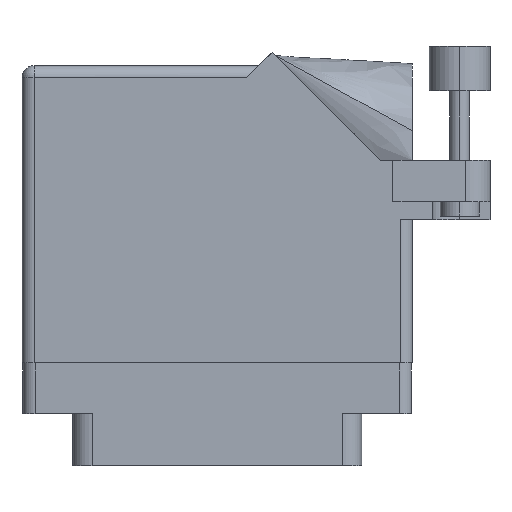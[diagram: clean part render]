
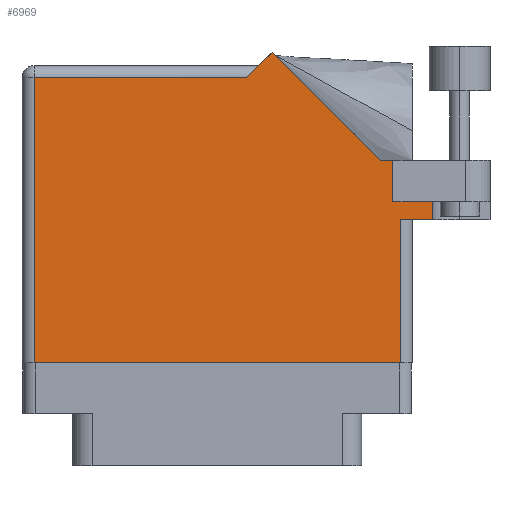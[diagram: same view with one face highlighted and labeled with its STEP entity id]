
A CAD part, front view. The second image highlights one B-rep face of the part: STEP entity #6969.
In plain terms, the highlighted face is planar.
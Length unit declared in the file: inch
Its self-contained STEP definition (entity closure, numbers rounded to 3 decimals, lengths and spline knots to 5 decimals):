
#476 = CARTESIAN_POINT ( 'NONE',  ( 2.1115, 1.16177, 0. ) ) ;
#520 = DIRECTION ( 'NONE',  ( 0., 1., 0. ) ) ;
#917 = CARTESIAN_POINT ( 'NONE',  ( 1.217, 1.53, 0. ) ) ;
#1288 = ORIENTED_EDGE ( 'NONE', *, *, #13473, .T. ) ;
#1426 = VECTOR ( 'NONE', #3656, 39.37008 ) ;
#2371 = ORIENTED_EDGE ( 'NONE', *, *, #24160, .T. ) ;
#2692 = VERTEX_POINT ( 'NONE', #9804 ) ;
#2951 = LINE ( 'NONE', #38883, #31933 ) ;
#3011 = DIRECTION ( 'NONE',  ( 1., 0., 0. ) ) ;
#3620 = VERTEX_POINT ( 'NONE', #18843 ) ;
#3656 = DIRECTION ( 'NONE',  ( -0.707, -0.707, 0. ) ) ;
#3920 = CARTESIAN_POINT ( 'NONE',  ( 1.84442, 1.044, 0. ) ) ;
#4170 = LINE ( 'NONE', #12082, #34573 ) ;
#4272 = VERTEX_POINT ( 'NONE', #17402 ) ;
#4332 = ORIENTED_EDGE ( 'NONE', *, *, #19496, .T. ) ;
#4532 = VECTOR ( 'NONE', #7852, 39.37008 ) ;
#5085 = EDGE_CURVE ( 'NONE', #17745, #25704, #18032, .T. ) ;
#6712 = VECTOR ( 'NONE', #9909, 39.37008 ) ;
#6969 = ADVANCED_FACE ( 'NONE', ( #23061 ), #28050, .F. ) ;
#7198 = ORIENTED_EDGE ( 'NONE', *, *, #5085, .T. ) ;
#7803 = CARTESIAN_POINT ( 'NONE',  ( 1.84442, 1.044, 0. ) ) ;
#7852 = DIRECTION ( 'NONE',  ( -1., 0., 0. ) ) ;
#8008 = DIRECTION ( 'NONE',  ( 0., -1., 0. ) ) ;
#8242 = EDGE_CURVE ( 'NONE', #23739, #4272, #24572, .T. ) ;
#9316 = VERTEX_POINT ( 'NONE', #32842 ) ;
#9490 = CARTESIAN_POINT ( 'NONE',  ( 0., 1.53, 0. ) ) ;
#9804 = CARTESIAN_POINT ( 'NONE',  ( 1.948, 0., 0. ) ) ;
#9883 = DIRECTION ( 'NONE',  ( 0., 0., -1. ) ) ;
#9909 = DIRECTION ( 'NONE',  ( 1., 0., 0. ) ) ;
#9930 = VECTOR ( 'NONE', #29068, 39.37008 ) ;
#10532 = CARTESIAN_POINT ( 'NONE',  ( 1.28771, 1.60071, 0. ) ) ;
#10705 = CARTESIAN_POINT ( 'NONE',  ( 0.062, 1.468, 0. ) ) ;
#11005 = ORIENTED_EDGE ( 'NONE', *, *, #18687, .F. ) ;
#11938 = VERTEX_POINT ( 'NONE', #29782 ) ;
#12082 = CARTESIAN_POINT ( 'NONE',  ( 1.91, 0.831, 0. ) ) ;
#12154 = ORIENTED_EDGE ( 'NONE', *, *, #19213, .T. ) ;
#12730 = LINE ( 'NONE', #22027, #35997 ) ;
#13073 = CARTESIAN_POINT ( 'NONE',  ( 2.01, 0.737, 0. ) ) ;
#13217 = CARTESIAN_POINT ( 'NONE',  ( 2.1115, 0.831, 0. ) ) ;
#13473 = EDGE_CURVE ( 'NONE', #11938, #17745, #15976, .T. ) ;
#14823 = DIRECTION ( 'NONE',  ( -1., 0., 0. ) ) ;
#15074 = ORIENTED_EDGE ( 'NONE', *, *, #16124, .T. ) ;
#15083 = LINE ( 'NONE', #32227, #33104 ) ;
#15620 = DIRECTION ( 'NONE',  ( 0., -1., 0. ) ) ;
#15976 = LINE ( 'NONE', #38513, #4532 ) ;
#16124 = EDGE_CURVE ( 'NONE', #2692, #9316, #2951, .T. ) ;
#16677 = EDGE_CURVE ( 'NONE', #30541, #2692, #30990, .T. ) ;
#16974 = VERTEX_POINT ( 'NONE', #10705 ) ;
#17124 = LINE ( 'NONE', #917, #1426 ) ;
#17402 = CARTESIAN_POINT ( 'NONE',  ( 2.1115, 0.737, 0. ) ) ;
#17731 = EDGE_CURVE ( 'NONE', #25704, #3620, #17124, .T. ) ;
#17745 = VERTEX_POINT ( 'NONE', #3920 ) ;
#17789 = LINE ( 'NONE', #13073, #22056 ) ;
#18032 = LINE ( 'NONE', #7803, #9930 ) ;
#18687 = EDGE_CURVE ( 'NONE', #32509, #23739, #4170, .T. ) ;
#18833 = EDGE_CURVE ( 'NONE', #32509, #11938, #12730, .T. ) ;
#18843 = CARTESIAN_POINT ( 'NONE',  ( 1.155, 1.468, 0. ) ) ;
#19213 = EDGE_CURVE ( 'NONE', #16974, #30541, #36444, .T. ) ;
#19496 = EDGE_CURVE ( 'NONE', #3620, #16974, #15083, .T. ) ;
#20102 = CARTESIAN_POINT ( 'NONE',  ( 0.062, 0., 0. ) ) ;
#20828 = ORIENTED_EDGE ( 'NONE', *, *, #8242, .F. ) ;
#22027 = CARTESIAN_POINT ( 'NONE',  ( 1.91, 0.831, 0. ) ) ;
#22056 = VECTOR ( 'NONE', #27670, 39.37008 ) ;
#23061 = FACE_OUTER_BOUND ( 'NONE', #38602, .T. ) ;
#23434 = CARTESIAN_POINT ( 'NONE',  ( 1.91, 0.831, 0. ) ) ;
#23739 = VERTEX_POINT ( 'NONE', #13217 ) ;
#24160 = EDGE_CURVE ( 'NONE', #9316, #4272, #17789, .T. ) ;
#24572 = LINE ( 'NONE', #476, #31721 ) ;
#24575 = VECTOR ( 'NONE', #8008, 39.37008 ) ;
#24699 = ORIENTED_EDGE ( 'NONE', *, *, #18833, .T. ) ;
#25704 = VERTEX_POINT ( 'NONE', #10532 ) ;
#26702 = DIRECTION ( 'NONE',  ( 0., 1., 0. ) ) ;
#27670 = DIRECTION ( 'NONE',  ( 1., 0., 0. ) ) ;
#27754 = CARTESIAN_POINT ( 'NONE',  ( 0.062, 0., 0. ) ) ;
#28050 = PLANE ( 'NONE',  #33389 ) ;
#29068 = DIRECTION ( 'NONE',  ( -0.707, 0.707, 0. ) ) ;
#29782 = CARTESIAN_POINT ( 'NONE',  ( 1.91, 1.044, 0. ) ) ;
#30541 = VERTEX_POINT ( 'NONE', #27754 ) ;
#30990 = LINE ( 'NONE', #37104, #6712 ) ;
#31132 = DIRECTION ( 'NONE',  ( -1., 0., 0. ) ) ;
#31156 = ORIENTED_EDGE ( 'NONE', *, *, #17731, .T. ) ;
#31613 = ORIENTED_EDGE ( 'NONE', *, *, #16677, .T. ) ;
#31721 = VECTOR ( 'NONE', #15620, 39.37008 ) ;
#31933 = VECTOR ( 'NONE', #26702, 39.37008 ) ;
#32227 = CARTESIAN_POINT ( 'NONE',  ( 0., 1.468, 0. ) ) ;
#32509 = VERTEX_POINT ( 'NONE', #23434 ) ;
#32842 = CARTESIAN_POINT ( 'NONE',  ( 1.948, 0.737, 0. ) ) ;
#33104 = VECTOR ( 'NONE', #14823, 39.37008 ) ;
#33389 = AXIS2_PLACEMENT_3D ( 'NONE', #9490, #9883, #31132 ) ;
#34573 = VECTOR ( 'NONE', #3011, 39.37008 ) ;
#35997 = VECTOR ( 'NONE', #520, 39.37008 ) ;
#36444 = LINE ( 'NONE', #20102, #24575 ) ;
#37104 = CARTESIAN_POINT ( 'NONE',  ( 0., 0., 0. ) ) ;
#38513 = CARTESIAN_POINT ( 'NONE',  ( 2.41, 1.044, 0. ) ) ;
#38602 = EDGE_LOOP ( 'NONE', ( #31613, #15074, #2371, #20828, #11005, #24699, #1288, #7198, #31156, #4332, #12154 ) ) ;
#38883 = CARTESIAN_POINT ( 'NONE',  ( 1.948, 0.737, 0. ) ) ;
